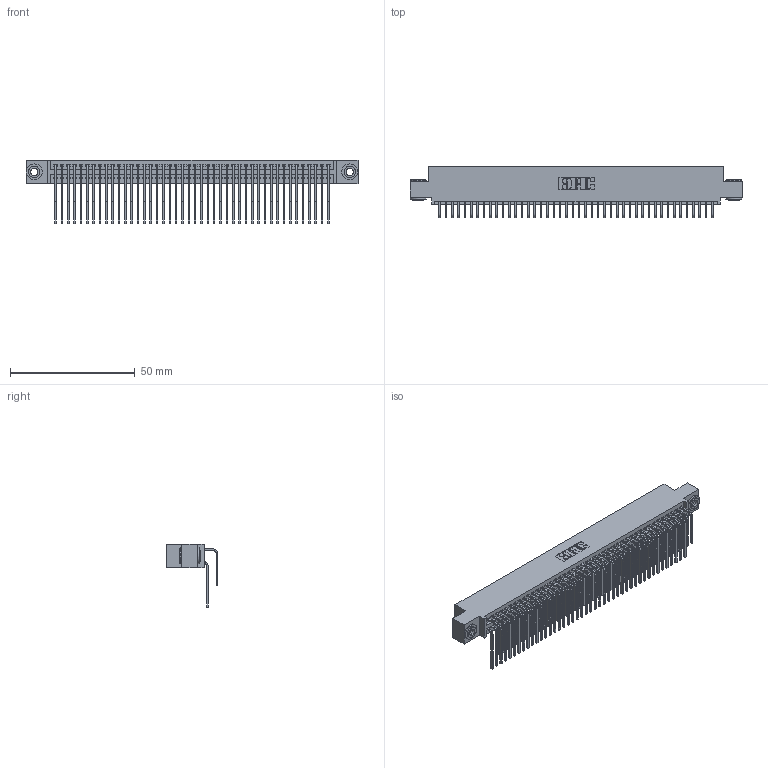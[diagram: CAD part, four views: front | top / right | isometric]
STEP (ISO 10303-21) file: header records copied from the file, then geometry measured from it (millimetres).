
FILE_DESCRIPTION (( 'STEP AP203' ), '1' );
FILE_NAME ('345-088-559-503.STEP', '2018-10-04T15:13:39', ( '' ), ( '' ), 'SwSTEP 2.0', 'SolidWorks 2016', '' );
FILE_SCHEMA (( 'CONFIG_CONTROL_DESIGN' ));
Length unit declared in the file: inch
Products named in the file (5): 345-088-559-503; 345-250-002_345-250-002-102; 345-292-001_558 559 Tail - 1; 345 Part_0.110 Offset - 0.156 Dia-TH; 345-292-001_559 Tail - 2
Assembly tree (91 placements, depth 2):
  345-088-559-503
    345 Part_0.110 Offset - 0.156 Dia-TH
    345-292-001_558 559 Tail - 1  x44
    345-292-001_559 Tail - 2  x44
    345-250-002_345-250-002-102  x2
Bounding box: 132.97 x 20.56 x 25.53 mm (x, y, z)
Volume: 13389 mm3; surface area: 22514.8 mm2
Topology: 91 solids, 91 shells, 4744 faces, 14069 edges, 9258 vertices
Faces by surface type: plane 3174, cylinder 1562, cone 8
Entity records: 36688 total; most frequent: CARTESIAN_POINT 6170, ORIENTED_EDGE 6046, DIRECTION 5441, EDGE_CURVE 3023, VECTOR 2651, LINE 2651, VERTEX_POINT 2010, AXIS2_PLACEMENT_3D 1395
